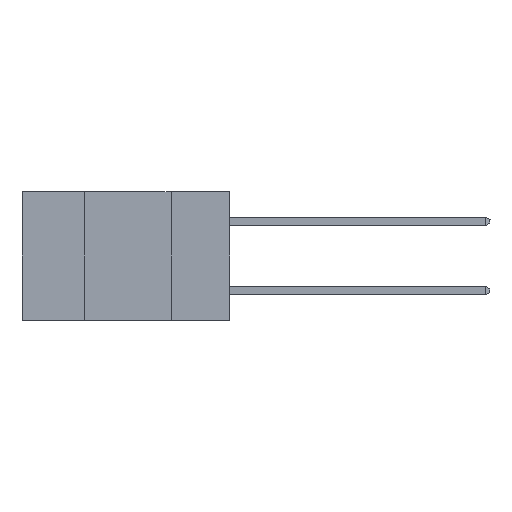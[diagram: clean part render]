
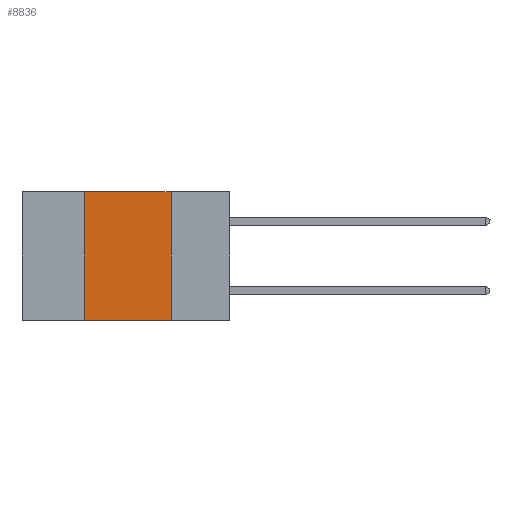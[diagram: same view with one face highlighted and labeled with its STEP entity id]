
A CAD part, left-side view. The second image highlights one B-rep face of the part: STEP entity #8836.
In plain terms, the highlighted planar face has unit normal (-1, 0, 0).
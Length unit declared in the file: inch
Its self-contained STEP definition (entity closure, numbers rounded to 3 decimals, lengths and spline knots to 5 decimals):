
#800 = VERTEX_POINT ( 'NONE', #3760 ) ;
#1338 = CARTESIAN_POINT ( 'NONE',  ( 0., 0.6, -0.37 ) ) ;
#1513 = AXIS2_PLACEMENT_3D ( 'NONE', #14304, #27788, #25656 ) ;
#2363 = VECTOR ( 'NONE', #8175, 39.37008 ) ;
#2832 = EDGE_LOOP ( 'NONE', ( #9961, #17378, #26490, #11870 ) ) ;
#3192 = VERTEX_POINT ( 'NONE', #18852 ) ;
#3760 = CARTESIAN_POINT ( 'NONE',  ( 0., 0.42, 0. ) ) ;
#4733 = LINE ( 'NONE', #26973, #23583 ) ;
#4985 = LINE ( 'NONE', #13058, #28676 ) ;
#8175 = DIRECTION ( 'NONE',  ( 0., -1., 0. ) ) ;
#8286 = VECTOR ( 'NONE', #15993, 39.37008 ) ;
#8836 = ADVANCED_FACE ( 'NONE', ( #11831 ), #12251, .F. ) ;
#9650 = EDGE_CURVE ( 'NONE', #16028, #3192, #18358, .T. ) ;
#9961 = ORIENTED_EDGE ( 'NONE', *, *, #9650, .F. ) ;
#11831 = FACE_OUTER_BOUND ( 'NONE', #2832, .T. ) ;
#11870 = ORIENTED_EDGE ( 'NONE', *, *, #19977, .T. ) ;
#12251 = PLANE ( 'NONE',  #1513 ) ;
#13058 = CARTESIAN_POINT ( 'NONE',  ( 0., 0.42, 0. ) ) ;
#13197 = LINE ( 'NONE', #1338, #2363 ) ;
#14304 = CARTESIAN_POINT ( 'NONE',  ( 0., 0.6, 0. ) ) ;
#15993 = DIRECTION ( 'NONE',  ( 0., 0., -1. ) ) ;
#16012 = DIRECTION ( 'NONE',  ( 0., -1., 0. ) ) ;
#16028 = VERTEX_POINT ( 'NONE', #28156 ) ;
#17378 = ORIENTED_EDGE ( 'NONE', *, *, #20986, .F. ) ;
#18358 = LINE ( 'NONE', #22487, #8286 ) ;
#18852 = CARTESIAN_POINT ( 'NONE',  ( 0., 0.17, -0.37 ) ) ;
#19977 = EDGE_CURVE ( 'NONE', #21919, #3192, #13197, .T. ) ;
#20986 = EDGE_CURVE ( 'NONE', #800, #16028, #4733, .T. ) ;
#21919 = VERTEX_POINT ( 'NONE', #26731 ) ;
#22487 = CARTESIAN_POINT ( 'NONE',  ( 0., 0.17, 0. ) ) ;
#23170 = EDGE_CURVE ( 'NONE', #21919, #800, #4985, .T. ) ;
#23583 = VECTOR ( 'NONE', #16012, 39.37008 ) ;
#25656 = DIRECTION ( 'NONE',  ( 0., 0., -1. ) ) ;
#26490 = ORIENTED_EDGE ( 'NONE', *, *, #23170, .F. ) ;
#26731 = CARTESIAN_POINT ( 'NONE',  ( 0., 0.42, -0.37 ) ) ;
#26973 = CARTESIAN_POINT ( 'NONE',  ( 0., 0.6, 0. ) ) ;
#27788 = DIRECTION ( 'NONE',  ( 1., 0., 0. ) ) ;
#28156 = CARTESIAN_POINT ( 'NONE',  ( 0., 0.17, 0. ) ) ;
#28589 = DIRECTION ( 'NONE',  ( 0., 0., 1. ) ) ;
#28676 = VECTOR ( 'NONE', #28589, 39.37008 ) ;
